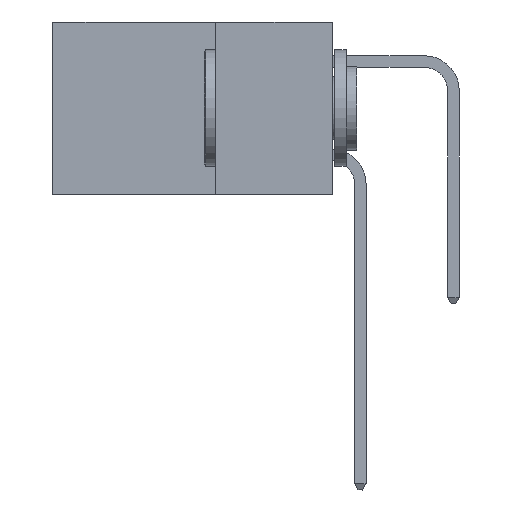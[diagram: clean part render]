
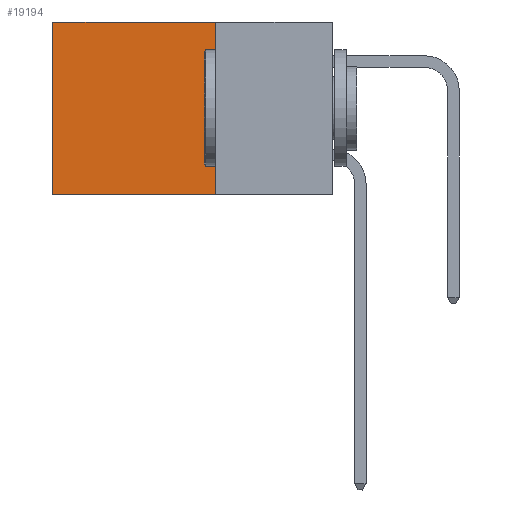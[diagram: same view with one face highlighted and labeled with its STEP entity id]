
A CAD part, left-side view. The second image highlights one B-rep face of the part: STEP entity #19194.
In plain terms, the highlighted planar face has unit normal (-1, 0, 0).
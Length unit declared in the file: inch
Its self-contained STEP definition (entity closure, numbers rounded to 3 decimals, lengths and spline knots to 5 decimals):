
#154 = VERTEX_POINT ( 'NONE', #12257 ) ;
#219 = CARTESIAN_POINT ( 'NONE',  ( 0.298, 0.25, 0. ) ) ;
#535 = VECTOR ( 'NONE', #13023, 39.37008 ) ;
#838 = CARTESIAN_POINT ( 'NONE',  ( 0.298, 0.25, 0. ) ) ;
#1310 = CARTESIAN_POINT ( 'NONE',  ( 0.298, 0.25, -0.37 ) ) ;
#2838 = LINE ( 'NONE', #1310, #18493 ) ;
#3459 = DIRECTION ( 'NONE',  ( 0., 1., 0. ) ) ;
#4712 = LINE ( 'NONE', #6697, #10331 ) ;
#5620 = VECTOR ( 'NONE', #26085, 39.37008 ) ;
#6178 = PLANE ( 'NONE',  #9806 ) ;
#6697 = CARTESIAN_POINT ( 'NONE',  ( 0.298, 0.6, 0. ) ) ;
#7156 = VERTEX_POINT ( 'NONE', #13175 ) ;
#9188 = ORIENTED_EDGE ( 'NONE', *, *, #12050, .F. ) ;
#9806 = AXIS2_PLACEMENT_3D ( 'NONE', #25097, #12608, #27147 ) ;
#10331 = VECTOR ( 'NONE', #21461, 39.37008 ) ;
#11211 = LINE ( 'NONE', #219, #535 ) ;
#11259 = LINE ( 'NONE', #11395, #5620 ) ;
#11395 = CARTESIAN_POINT ( 'NONE',  ( 0.298, 0.25, 0. ) ) ;
#12050 = EDGE_CURVE ( 'NONE', #22555, #7156, #11259, .T. ) ;
#12257 = CARTESIAN_POINT ( 'NONE',  ( 0.298, 0.6, -0.37 ) ) ;
#12608 = DIRECTION ( 'NONE',  ( 1., 0., 0. ) ) ;
#13023 = DIRECTION ( 'NONE',  ( 0., 1., 0. ) ) ;
#13175 = CARTESIAN_POINT ( 'NONE',  ( 0.298, 0.25, -0.37 ) ) ;
#13637 = EDGE_LOOP ( 'NONE', ( #20594, #24770, #9188, #25833 ) ) ;
#17373 = FACE_OUTER_BOUND ( 'NONE', #13637, .T. ) ;
#18493 = VECTOR ( 'NONE', #3459, 39.37008 ) ;
#19194 = ADVANCED_FACE ( 'NONE', ( #17373 ), #6178, .F. ) ;
#19755 = EDGE_CURVE ( 'NONE', #25594, #154, #4712, .T. ) ;
#20594 = ORIENTED_EDGE ( 'NONE', *, *, #19755, .T. ) ;
#21461 = DIRECTION ( 'NONE',  ( 0., 0., -1. ) ) ;
#21580 = CARTESIAN_POINT ( 'NONE',  ( 0.298, 0.6, 0. ) ) ;
#21678 = EDGE_CURVE ( 'NONE', #22555, #25594, #11211, .T. ) ;
#22555 = VERTEX_POINT ( 'NONE', #838 ) ;
#23357 = EDGE_CURVE ( 'NONE', #7156, #154, #2838, .T. ) ;
#24770 = ORIENTED_EDGE ( 'NONE', *, *, #23357, .F. ) ;
#25097 = CARTESIAN_POINT ( 'NONE',  ( 0.298, 0.25, 0. ) ) ;
#25594 = VERTEX_POINT ( 'NONE', #21580 ) ;
#25833 = ORIENTED_EDGE ( 'NONE', *, *, #21678, .T. ) ;
#26085 = DIRECTION ( 'NONE',  ( 0., 0., -1. ) ) ;
#27147 = DIRECTION ( 'NONE',  ( 0., 0., -1. ) ) ;
